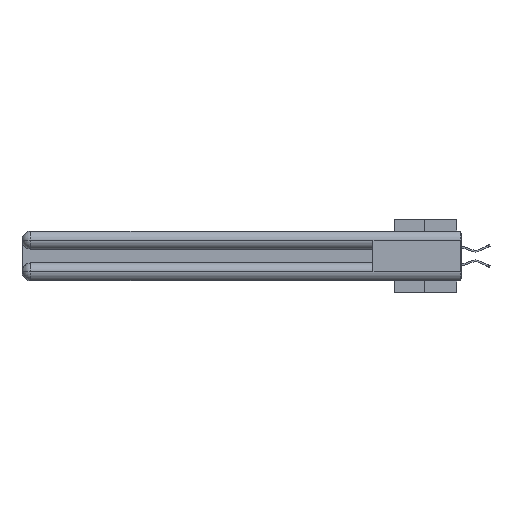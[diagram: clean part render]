
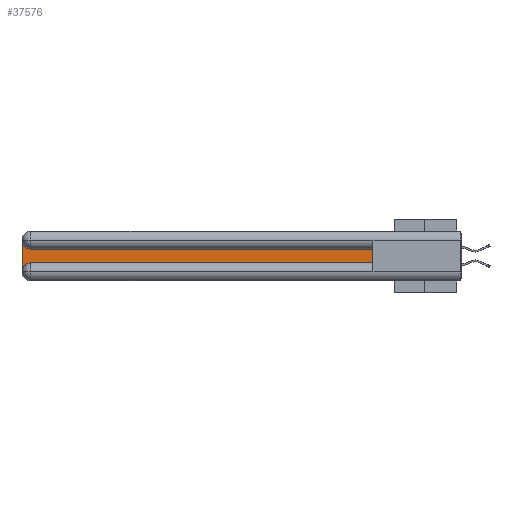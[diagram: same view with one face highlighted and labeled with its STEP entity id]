
A CAD part, left-side view. The second image highlights one B-rep face of the part: STEP entity #37576.
In plain terms, the highlighted planar face has unit normal (-1, 0, 0).
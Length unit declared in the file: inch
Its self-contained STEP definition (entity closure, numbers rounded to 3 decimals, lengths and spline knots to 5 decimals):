
#1405 = EDGE_LOOP ( 'NONE', ( #20356, #2081, #11157, #29012, #17455, #18774 ) ) ;
#1784 = CARTESIAN_POINT ( 'NONE',  ( 0.075, 2.94, -0.0625 ) ) ;
#1829 = CARTESIAN_POINT ( 'NONE',  ( 0.075, 2.94, -0.1225 ) ) ;
#2027 = VECTOR ( 'NONE', #16623, 39.37008 ) ;
#2081 = ORIENTED_EDGE ( 'NONE', *, *, #7456, .T. ) ;
#4233 = VECTOR ( 'NONE', #18607, 39.37008 ) ;
#4781 = PLANE ( 'NONE',  #21748 ) ;
#7076 = CARTESIAN_POINT ( 'NONE',  ( 0.075, 3., -0.0625 ) ) ;
#7321 = AXIS2_PLACEMENT_3D ( 'NONE', #25437, #28589, #31791 ) ;
#7332 = VERTEX_POINT ( 'NONE', #33758 ) ;
#7456 = EDGE_CURVE ( 'NONE', #29105, #32690, #36295, .T. ) ;
#7779 = LINE ( 'NONE', #19828, #34774 ) ;
#9926 = CARTESIAN_POINT ( 'NONE',  ( 0.075, 3., -0.2175 ) ) ;
#10743 = CARTESIAN_POINT ( 'NONE',  ( 0.075, 0.6, -0.2175 ) ) ;
#11157 = ORIENTED_EDGE ( 'NONE', *, *, #21895, .T. ) ;
#11193 = VERTEX_POINT ( 'NONE', #24440 ) ;
#12364 = LINE ( 'NONE', #9926, #2027 ) ;
#14078 = DIRECTION ( 'NONE',  ( 1., 0., 0. ) ) ;
#15077 = EDGE_CURVE ( 'NONE', #7332, #15742, #24077, .T. ) ;
#15742 = VERTEX_POINT ( 'NONE', #26542 ) ;
#16623 = DIRECTION ( 'NONE',  ( 0., 0., -1. ) ) ;
#16828 = DIRECTION ( 'NONE',  ( 0., 1., 0. ) ) ;
#17171 = EDGE_CURVE ( 'NONE', #34766, #7332, #20086, .T. ) ;
#17414 = DIRECTION ( 'NONE',  ( 0., 0., -1. ) ) ;
#17455 = ORIENTED_EDGE ( 'NONE', *, *, #15077, .T. ) ;
#18320 = FACE_OUTER_BOUND ( 'NONE', #1405, .T. ) ;
#18607 = DIRECTION ( 'NONE',  ( 0., 0., 1. ) ) ;
#18774 = ORIENTED_EDGE ( 'NONE', *, *, #19019, .T. ) ;
#19019 = EDGE_CURVE ( 'NONE', #15742, #11193, #32238, .T. ) ;
#19828 = CARTESIAN_POINT ( 'NONE',  ( 0.075, 0.6, -0.1225 ) ) ;
#20086 = CIRCLE ( 'NONE', #7321, 0.06 ) ;
#20356 = ORIENTED_EDGE ( 'NONE', *, *, #40474, .T. ) ;
#21748 = AXIS2_PLACEMENT_3D ( 'NONE', #23116, #14078, #36150 ) ;
#21895 = EDGE_CURVE ( 'NONE', #32690, #34766, #12364, .T. ) ;
#23116 = CARTESIAN_POINT ( 'NONE',  ( 0.075, 3., -0.1225 ) ) ;
#24077 = LINE ( 'NONE', #10743, #27007 ) ;
#24440 = CARTESIAN_POINT ( 'NONE',  ( 0.075, 0.6, -0.1225 ) ) ;
#25437 = CARTESIAN_POINT ( 'NONE',  ( 0.075, 2.94, -0.2775 ) ) ;
#26542 = CARTESIAN_POINT ( 'NONE',  ( 0.075, 0.6, -0.2175 ) ) ;
#27007 = VECTOR ( 'NONE', #32697, 39.37008 ) ;
#28589 = DIRECTION ( 'NONE',  ( 1., 0., 0. ) ) ;
#29012 = ORIENTED_EDGE ( 'NONE', *, *, #17171, .T. ) ;
#29105 = VERTEX_POINT ( 'NONE', #1829 ) ;
#31791 = DIRECTION ( 'NONE',  ( 0., 0., -1. ) ) ;
#32238 = LINE ( 'NONE', #37395, #4233 ) ;
#32690 = VERTEX_POINT ( 'NONE', #7076 ) ;
#32697 = DIRECTION ( 'NONE',  ( 0., -1., 0. ) ) ;
#33491 = DIRECTION ( 'NONE',  ( 1., 0., 0. ) ) ;
#33758 = CARTESIAN_POINT ( 'NONE',  ( 0.075, 2.94, -0.2175 ) ) ;
#33937 = CARTESIAN_POINT ( 'NONE',  ( 0.075, 3., -0.2775 ) ) ;
#34766 = VERTEX_POINT ( 'NONE', #33937 ) ;
#34774 = VECTOR ( 'NONE', #16828, 39.37008 ) ;
#36150 = DIRECTION ( 'NONE',  ( 0., 0., -1. ) ) ;
#36295 = CIRCLE ( 'NONE', #38438, 0.06 ) ;
#37395 = CARTESIAN_POINT ( 'NONE',  ( 0.075, 0.6, -0.2175 ) ) ;
#37576 = ADVANCED_FACE ( 'NONE', ( #18320 ), #4781, .F. ) ;
#38438 = AXIS2_PLACEMENT_3D ( 'NONE', #1784, #33491, #17414 ) ;
#40474 = EDGE_CURVE ( 'NONE', #11193, #29105, #7779, .T. ) ;
